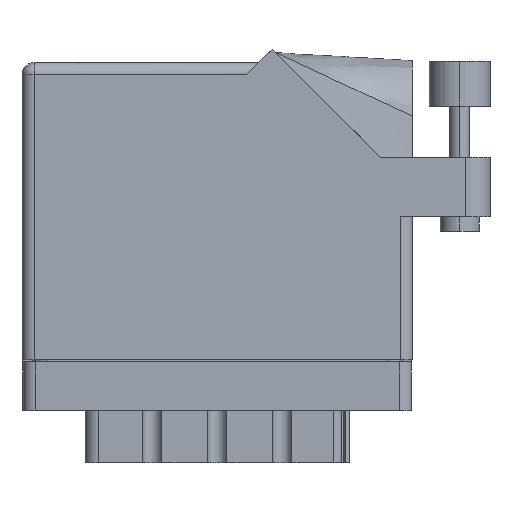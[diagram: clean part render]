
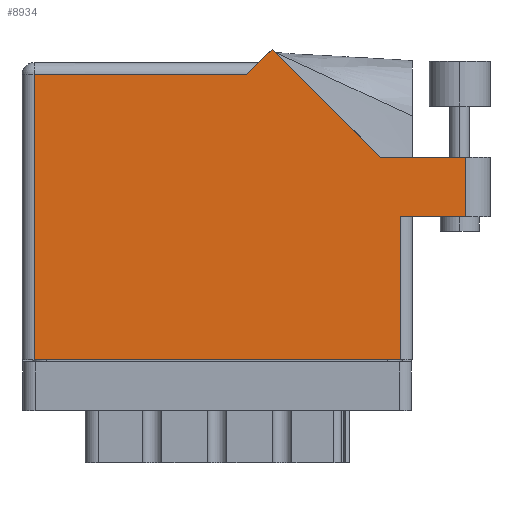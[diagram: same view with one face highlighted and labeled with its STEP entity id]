
A CAD part, front view. The second image highlights one B-rep face of the part: STEP entity #8934.
In plain terms, the highlighted face is planar.
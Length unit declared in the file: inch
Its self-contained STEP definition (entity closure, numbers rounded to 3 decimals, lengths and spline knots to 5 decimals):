
#152 = CARTESIAN_POINT ( 'NONE',  ( 2.285, 1.044, 0. ) ) ;
#1401 = CARTESIAN_POINT ( 'NONE',  ( 2.285, 1.044, 0. ) ) ;
#1925 = CARTESIAN_POINT ( 'NONE',  ( 1.84442, 1.044, 0. ) ) ;
#2177 = CARTESIAN_POINT ( 'NONE',  ( 1.948, 0.737, 0. ) ) ;
#2464 = ORIENTED_EDGE ( 'NONE', *, *, #11834, .T. ) ;
#3020 = VERTEX_POINT ( 'NONE', #2177 ) ;
#3060 = AXIS2_PLACEMENT_3D ( 'NONE', #15613, #9853, #35517 ) ;
#3747 = CARTESIAN_POINT ( 'NONE',  ( 0.062, 1.468, 0. ) ) ;
#4134 = VECTOR ( 'NONE', #11927, 39.37008 ) ;
#5951 = DIRECTION ( 'NONE',  ( 1., 0., 0. ) ) ;
#6098 = LINE ( 'NONE', #9520, #24050 ) ;
#7029 = VERTEX_POINT ( 'NONE', #9067 ) ;
#7858 = CARTESIAN_POINT ( 'NONE',  ( 2.285, 0.737, 0. ) ) ;
#7882 = EDGE_LOOP ( 'NONE', ( #12547, #29406, #8430, #22015, #24947, #34764, #2464, #11368, #21288 ) ) ;
#8430 = ORIENTED_EDGE ( 'NONE', *, *, #25481, .T. ) ;
#8501 = VECTOR ( 'NONE', #5951, 39.37008 ) ;
#8704 = CARTESIAN_POINT ( 'NONE',  ( 1.948, 0.737, 0. ) ) ;
#8934 = ADVANCED_FACE ( 'NONE', ( #31852 ), #15365, .F. ) ;
#9067 = CARTESIAN_POINT ( 'NONE',  ( 1.948, 0., 0. ) ) ;
#9174 = VECTOR ( 'NONE', #12244, 39.37008 ) ;
#9520 = CARTESIAN_POINT ( 'NONE',  ( 1.84442, 1.044, 0. ) ) ;
#9563 = LINE ( 'NONE', #14935, #4134 ) ;
#9853 = DIRECTION ( 'NONE',  ( 0., 0., -1. ) ) ;
#10101 = LINE ( 'NONE', #152, #28964 ) ;
#11130 = VERTEX_POINT ( 'NONE', #1401 ) ;
#11244 = CARTESIAN_POINT ( 'NONE',  ( 2.01, 0.737, 0. ) ) ;
#11368 = ORIENTED_EDGE ( 'NONE', *, *, #34193, .T. ) ;
#11834 = EDGE_CURVE ( 'NONE', #29785, #29732, #22679, .T. ) ;
#11927 = DIRECTION ( 'NONE',  ( 1., 0., 0. ) ) ;
#12083 = CARTESIAN_POINT ( 'NONE',  ( 0.062, 0., 0. ) ) ;
#12119 = LINE ( 'NONE', #11244, #8501 ) ;
#12244 = DIRECTION ( 'NONE',  ( -0.707, -0.707, 0. ) ) ;
#12547 = ORIENTED_EDGE ( 'NONE', *, *, #28216, .T. ) ;
#12828 = DIRECTION ( 'NONE',  ( -1., 0., 0. ) ) ;
#13155 = DIRECTION ( 'NONE',  ( -0.707, 0.707, 0. ) ) ;
#13999 = EDGE_CURVE ( 'NONE', #7029, #3020, #24730, .T. ) ;
#14935 = CARTESIAN_POINT ( 'NONE',  ( 0., 0., 0. ) ) ;
#15365 = PLANE ( 'NONE',  #3060 ) ;
#15613 = CARTESIAN_POINT ( 'NONE',  ( 0., 1.53, 0. ) ) ;
#17201 = LINE ( 'NONE', #33183, #28841 ) ;
#18640 = LINE ( 'NONE', #29441, #9174 ) ;
#18914 = DIRECTION ( 'NONE',  ( -1., 0., 0. ) ) ;
#19096 = EDGE_CURVE ( 'NONE', #34393, #29785, #26566, .T. ) ;
#19310 = CARTESIAN_POINT ( 'NONE',  ( 1.155, 1.468, 0. ) ) ;
#21288 = ORIENTED_EDGE ( 'NONE', *, *, #13999, .T. ) ;
#21906 = CARTESIAN_POINT ( 'NONE',  ( 0., 1.468, 0. ) ) ;
#22015 = ORIENTED_EDGE ( 'NONE', *, *, #32605, .T. ) ;
#22018 = VECTOR ( 'NONE', #28803, 39.37008 ) ;
#22679 = LINE ( 'NONE', #34086, #29445 ) ;
#22917 = VERTEX_POINT ( 'NONE', #36515 ) ;
#24050 = VECTOR ( 'NONE', #13155, 39.37008 ) ;
#24730 = LINE ( 'NONE', #8704, #22018 ) ;
#24947 = ORIENTED_EDGE ( 'NONE', *, *, #30810, .T. ) ;
#25481 = EDGE_CURVE ( 'NONE', #11130, #32680, #17201, .T. ) ;
#26566 = LINE ( 'NONE', #21906, #32911 ) ;
#28216 = EDGE_CURVE ( 'NONE', #3020, #32686, #12119, .T. ) ;
#28701 = DIRECTION ( 'NONE',  ( 0., 1., 0. ) ) ;
#28803 = DIRECTION ( 'NONE',  ( 0., 1., 0. ) ) ;
#28841 = VECTOR ( 'NONE', #12828, 39.37008 ) ;
#28964 = VECTOR ( 'NONE', #28701, 39.37008 ) ;
#29406 = ORIENTED_EDGE ( 'NONE', *, *, #30699, .T. ) ;
#29441 = CARTESIAN_POINT ( 'NONE',  ( 1.217, 1.53, 0. ) ) ;
#29445 = VECTOR ( 'NONE', #37235, 39.37008 ) ;
#29732 = VERTEX_POINT ( 'NONE', #12083 ) ;
#29785 = VERTEX_POINT ( 'NONE', #3747 ) ;
#30699 = EDGE_CURVE ( 'NONE', #32686, #11130, #10101, .T. ) ;
#30810 = EDGE_CURVE ( 'NONE', #22917, #34393, #18640, .T. ) ;
#31852 = FACE_OUTER_BOUND ( 'NONE', #7882, .T. ) ;
#32605 = EDGE_CURVE ( 'NONE', #32680, #22917, #6098, .T. ) ;
#32680 = VERTEX_POINT ( 'NONE', #1925 ) ;
#32686 = VERTEX_POINT ( 'NONE', #7858 ) ;
#32911 = VECTOR ( 'NONE', #18914, 39.37008 ) ;
#33183 = CARTESIAN_POINT ( 'NONE',  ( 2.41, 1.044, 0. ) ) ;
#34086 = CARTESIAN_POINT ( 'NONE',  ( 0.062, 0., 0. ) ) ;
#34193 = EDGE_CURVE ( 'NONE', #29732, #7029, #9563, .T. ) ;
#34393 = VERTEX_POINT ( 'NONE', #19310 ) ;
#34764 = ORIENTED_EDGE ( 'NONE', *, *, #19096, .T. ) ;
#35517 = DIRECTION ( 'NONE',  ( -1., 0., 0. ) ) ;
#36515 = CARTESIAN_POINT ( 'NONE',  ( 1.28771, 1.60071, 0. ) ) ;
#37235 = DIRECTION ( 'NONE',  ( 0., -1., 0. ) ) ;
